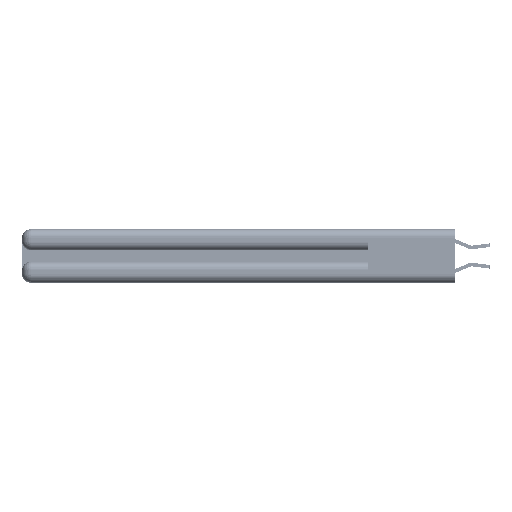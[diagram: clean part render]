
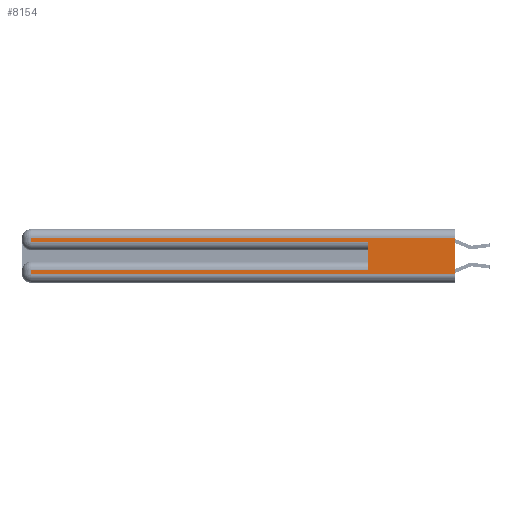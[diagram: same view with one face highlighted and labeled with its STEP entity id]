
A CAD part, left-side view. The second image highlights one B-rep face of the part: STEP entity #8154.
In plain terms, the highlighted planar face has unit normal (-1, 0, 0).
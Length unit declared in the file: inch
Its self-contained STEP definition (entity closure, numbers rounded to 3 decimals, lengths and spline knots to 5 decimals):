
#123 = CARTESIAN_POINT ( 'NONE',  ( 0., 0., 0.37 ) ) ;
#437 = DIRECTION ( 'NONE',  ( 0., 0., 1. ) ) ;
#1000 = VECTOR ( 'NONE', #31738, 39.37008 ) ;
#1238 = EDGE_CURVE ( 'NONE', #1992, #22319, #7922, .T. ) ;
#1896 = EDGE_CURVE ( 'NONE', #12102, #36150, #14876, .T. ) ;
#1912 = VERTEX_POINT ( 'NONE', #31192 ) ;
#1992 = VERTEX_POINT ( 'NONE', #31053 ) ;
#2006 = CARTESIAN_POINT ( 'NONE',  ( 0., 0.6, 0.085 ) ) ;
#3922 = LINE ( 'NONE', #5573, #16754 ) ;
#4358 = LINE ( 'NONE', #29421, #6113 ) ;
#5175 = DIRECTION ( 'NONE',  ( 0., 0., -1. ) ) ;
#5297 = VERTEX_POINT ( 'NONE', #30503 ) ;
#5417 = CARTESIAN_POINT ( 'NONE',  ( 0., 0., 0.37 ) ) ;
#5573 = CARTESIAN_POINT ( 'NONE',  ( 0., 0., 0.285 ) ) ;
#5575 = AXIS2_PLACEMENT_3D ( 'NONE', #123, #35432, #18569 ) ;
#6113 = VECTOR ( 'NONE', #15561, 39.37008 ) ;
#6394 = CARTESIAN_POINT ( 'NONE',  ( 0., 0., 0.06 ) ) ;
#7287 = LINE ( 'NONE', #13340, #17810 ) ;
#7865 = ORIENTED_EDGE ( 'NONE', *, *, #1896, .F. ) ;
#7922 = LINE ( 'NONE', #30867, #18008 ) ;
#8154 = ADVANCED_FACE ( 'NONE', ( #13582 ), #21081, .F. ) ;
#8257 = CARTESIAN_POINT ( 'NONE',  ( 0., 2.94, 0.285 ) ) ;
#8295 = VECTOR ( 'NONE', #26788, 39.37008 ) ;
#8822 = EDGE_CURVE ( 'NONE', #5297, #9033, #10029, .T. ) ;
#9033 = VERTEX_POINT ( 'NONE', #8257 ) ;
#9674 = ORIENTED_EDGE ( 'NONE', *, *, #30626, .T. ) ;
#9808 = ORIENTED_EDGE ( 'NONE', *, *, #20965, .T. ) ;
#10029 = LINE ( 'NONE', #18895, #8295 ) ;
#11418 = CARTESIAN_POINT ( 'NONE',  ( 0., 0.6, 0.145 ) ) ;
#12102 = VERTEX_POINT ( 'NONE', #2006 ) ;
#13340 = CARTESIAN_POINT ( 'NONE',  ( 0., 0., 0.31 ) ) ;
#13582 = FACE_OUTER_BOUND ( 'NONE', #30727, .T. ) ;
#14184 = DIRECTION ( 'NONE',  ( 0., 1., 0. ) ) ;
#14613 = DIRECTION ( 'NONE',  ( 0., -1., 0. ) ) ;
#14876 = LINE ( 'NONE', #11418, #15786 ) ;
#15127 = LINE ( 'NONE', #5417, #26662 ) ;
#15343 = EDGE_CURVE ( 'NONE', #1912, #22319, #15127, .T. ) ;
#15561 = DIRECTION ( 'NONE',  ( 0., 1., 0. ) ) ;
#15786 = VECTOR ( 'NONE', #437, 39.37008 ) ;
#16754 = VECTOR ( 'NONE', #28273, 39.37008 ) ;
#17761 = ORIENTED_EDGE ( 'NONE', *, *, #15343, .F. ) ;
#17810 = VECTOR ( 'NONE', #14184, 39.37008 ) ;
#18008 = VECTOR ( 'NONE', #14613, 39.37008 ) ;
#18569 = DIRECTION ( 'NONE',  ( 0., 0., -1. ) ) ;
#18895 = CARTESIAN_POINT ( 'NONE',  ( 0., 2.94, 0.37 ) ) ;
#19082 = ORIENTED_EDGE ( 'NONE', *, *, #8822, .T. ) ;
#20083 = CARTESIAN_POINT ( 'NONE',  ( 0., 2.94, 0.37 ) ) ;
#20965 = EDGE_CURVE ( 'NONE', #36458, #1992, #36359, .T. ) ;
#21081 = PLANE ( 'NONE',  #5575 ) ;
#22319 = VERTEX_POINT ( 'NONE', #6394 ) ;
#23922 = EDGE_CURVE ( 'NONE', #12102, #36458, #4358, .T. ) ;
#26662 = VECTOR ( 'NONE', #5175, 39.37008 ) ;
#26788 = DIRECTION ( 'NONE',  ( 0., 0., -1. ) ) ;
#28128 = ORIENTED_EDGE ( 'NONE', *, *, #1238, .T. ) ;
#28273 = DIRECTION ( 'NONE',  ( 0., -1., 0. ) ) ;
#29421 = CARTESIAN_POINT ( 'NONE',  ( 0., 0., 0.085 ) ) ;
#30503 = CARTESIAN_POINT ( 'NONE',  ( 0., 2.94, 0.31 ) ) ;
#30626 = EDGE_CURVE ( 'NONE', #9033, #36150, #3922, .T. ) ;
#30727 = EDGE_LOOP ( 'NONE', ( #17761, #33023, #19082, #9674, #7865, #34988, #9808, #28128 ) ) ;
#30867 = CARTESIAN_POINT ( 'NONE',  ( 0., 0., 0.06 ) ) ;
#31053 = CARTESIAN_POINT ( 'NONE',  ( 0., 2.94, 0.06 ) ) ;
#31192 = CARTESIAN_POINT ( 'NONE',  ( 0., 0., 0.31 ) ) ;
#31738 = DIRECTION ( 'NONE',  ( 0., 0., -1. ) ) ;
#32212 = CARTESIAN_POINT ( 'NONE',  ( 0., 2.94, 0.085 ) ) ;
#33023 = ORIENTED_EDGE ( 'NONE', *, *, #33136, .T. ) ;
#33136 = EDGE_CURVE ( 'NONE', #1912, #5297, #7287, .T. ) ;
#33969 = CARTESIAN_POINT ( 'NONE',  ( 0., 0.6, 0.285 ) ) ;
#34988 = ORIENTED_EDGE ( 'NONE', *, *, #23922, .T. ) ;
#35432 = DIRECTION ( 'NONE',  ( 1., 0., 0. ) ) ;
#36150 = VERTEX_POINT ( 'NONE', #33969 ) ;
#36359 = LINE ( 'NONE', #20083, #1000 ) ;
#36458 = VERTEX_POINT ( 'NONE', #32212 ) ;
